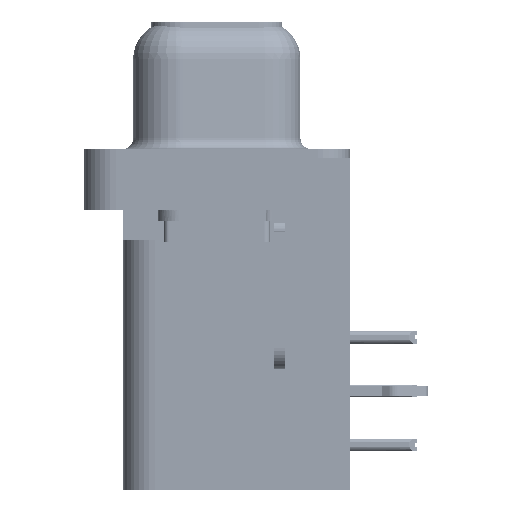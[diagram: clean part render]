
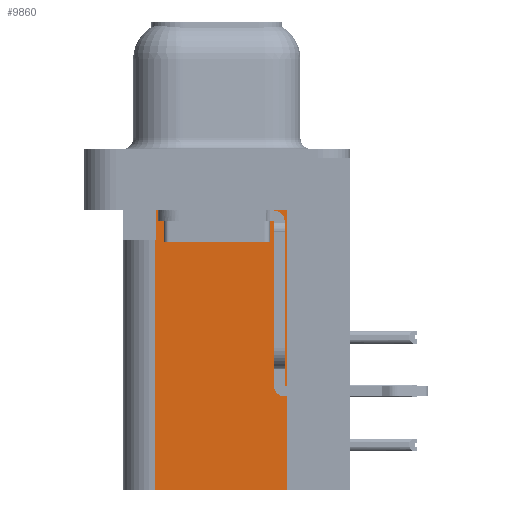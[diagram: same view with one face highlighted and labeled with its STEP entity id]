
A CAD part, left-side view. The second image highlights one B-rep face of the part: STEP entity #9860.
In plain terms, the highlighted planar face has unit normal (-1, 0, 0).
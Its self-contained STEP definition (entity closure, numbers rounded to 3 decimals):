
#824 = CARTESIAN_POINT ( 'NONE',  ( 3.79, 0., -3.9 ) ) ;
#1763 = EDGE_CURVE ( 'NONE', #20601, #32177, #7003, .T. ) ;
#6302 = EDGE_CURVE ( 'NONE', #38730, #19076, #52446, .T. ) ;
#6603 = CARTESIAN_POINT ( 'NONE',  ( 3.79, 2.895, -3.9 ) ) ;
#7003 = LINE ( 'NONE', #13812, #27587 ) ;
#7633 = CARTESIAN_POINT ( 'NONE',  ( 3.79, -3.295, -2.5 ) ) ;
#9860 = ADVANCED_FACE ( 'NONE', ( #46377 ), #47539, .F. ) ;
#10923 = ORIENTED_EDGE ( 'NONE', *, *, #30576, .T. ) ;
#13812 = CARTESIAN_POINT ( 'NONE',  ( 3.79, -3.295, -15.7 ) ) ;
#14088 = CARTESIAN_POINT ( 'NONE',  ( 3.79, 2.895, -3.9 ) ) ;
#15642 = VECTOR ( 'NONE', #23233, 1000. ) ;
#16318 = EDGE_CURVE ( 'NONE', #32177, #19076, #38674, .T. ) ;
#16915 = ORIENTED_EDGE ( 'NONE', *, *, #6302, .T. ) ;
#17905 = DIRECTION ( 'NONE',  ( 0., 1., 0. ) ) ;
#17989 = CARTESIAN_POINT ( 'NONE',  ( 3.79, -3.295, -15.7 ) ) ;
#18083 = VECTOR ( 'NONE', #50737, 1000. ) ;
#18735 = CARTESIAN_POINT ( 'NONE',  ( 3.79, 2.925, -3.9 ) ) ;
#19076 = VERTEX_POINT ( 'NONE', #18735 ) ;
#19244 = CARTESIAN_POINT ( 'NONE',  ( 3.79, -3.295, -15.7 ) ) ;
#19422 = DIRECTION ( 'NONE',  ( 0., 0., -1. ) ) ;
#20601 = VERTEX_POINT ( 'NONE', #34628 ) ;
#21185 = CARTESIAN_POINT ( 'NONE',  ( 3.79, 2.895, -2.5 ) ) ;
#21515 = ORIENTED_EDGE ( 'NONE', *, *, #16318, .F. ) ;
#22282 = LINE ( 'NONE', #14088, #30604 ) ;
#23233 = DIRECTION ( 'NONE',  ( 0., 0., 1. ) ) ;
#24031 = DIRECTION ( 'NONE',  ( 0., 1., 0. ) ) ;
#27357 = CARTESIAN_POINT ( 'NONE',  ( 3.79, 2.925, -15.7 ) ) ;
#27587 = VECTOR ( 'NONE', #17905, 1000. ) ;
#30576 = EDGE_CURVE ( 'NONE', #41739, #38730, #22282, .T. ) ;
#30604 = VECTOR ( 'NONE', #42504, 1000. ) ;
#32177 = VERTEX_POINT ( 'NONE', #50396 ) ;
#33360 = EDGE_CURVE ( 'NONE', #35531, #41739, #49519, .T. ) ;
#34628 = CARTESIAN_POINT ( 'NONE',  ( 3.79, -3.295, -15.7 ) ) ;
#35483 = ORIENTED_EDGE ( 'NONE', *, *, #1763, .F. ) ;
#35531 = VERTEX_POINT ( 'NONE', #7633 ) ;
#35706 = AXIS2_PLACEMENT_3D ( 'NONE', #19244, #43923, #19422 ) ;
#38674 = LINE ( 'NONE', #27357, #15642 ) ;
#38730 = VERTEX_POINT ( 'NONE', #6603 ) ;
#38802 = ORIENTED_EDGE ( 'NONE', *, *, #33360, .T. ) ;
#39019 = VECTOR ( 'NONE', #50104, 1000. ) ;
#39898 = VECTOR ( 'NONE', #24031, 1000. ) ;
#41739 = VERTEX_POINT ( 'NONE', #21185 ) ;
#42504 = DIRECTION ( 'NONE',  ( 0., 0., -1. ) ) ;
#43741 = EDGE_CURVE ( 'NONE', #20601, #35531, #51982, .T. ) ;
#43923 = DIRECTION ( 'NONE',  ( 1., 0., 0. ) ) ;
#45381 = EDGE_LOOP ( 'NONE', ( #38802, #10923, #16915, #21515, #35483, #47191 ) ) ;
#46377 = FACE_OUTER_BOUND ( 'NONE', #45381, .T. ) ;
#47191 = ORIENTED_EDGE ( 'NONE', *, *, #43741, .T. ) ;
#47539 = PLANE ( 'NONE',  #35706 ) ;
#49519 = LINE ( 'NONE', #52611, #39898 ) ;
#50104 = DIRECTION ( 'NONE',  ( 0., 1., 0. ) ) ;
#50396 = CARTESIAN_POINT ( 'NONE',  ( 3.79, 2.925, -15.7 ) ) ;
#50737 = DIRECTION ( 'NONE',  ( 0., 0., 1. ) ) ;
#51982 = LINE ( 'NONE', #17989, #18083 ) ;
#52446 = LINE ( 'NONE', #824, #39019 ) ;
#52611 = CARTESIAN_POINT ( 'NONE',  ( 3.79, -3.295, -2.5 ) ) ;
